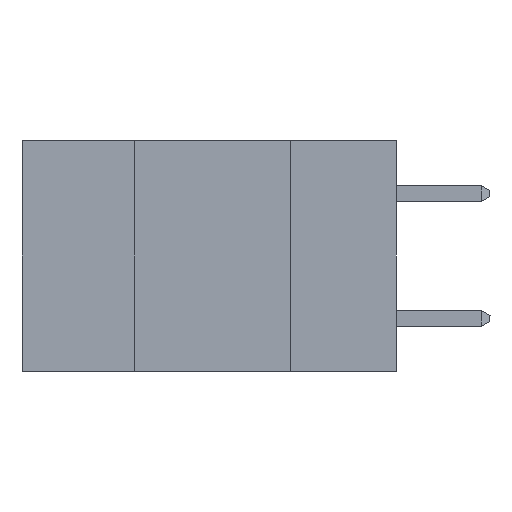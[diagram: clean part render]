
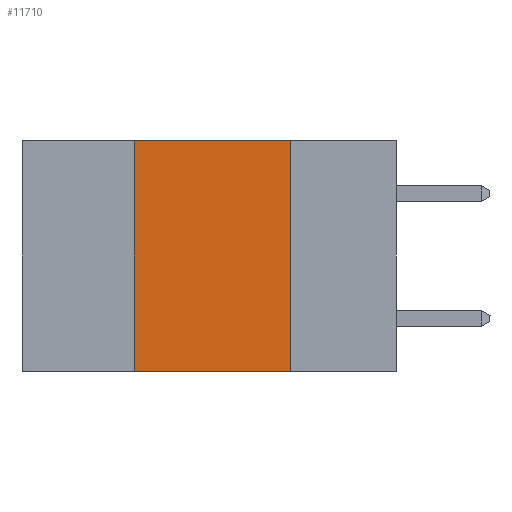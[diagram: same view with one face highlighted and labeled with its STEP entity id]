
A CAD part, left-side view. The second image highlights one B-rep face of the part: STEP entity #11710.
In plain terms, the highlighted planar face has unit normal (-1, 0, 0).
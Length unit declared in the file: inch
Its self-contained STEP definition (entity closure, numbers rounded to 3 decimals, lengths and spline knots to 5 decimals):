
#12 = ORIENTED_EDGE ( 'NONE', *, *, #7438, .F. ) ;
#440 = VECTOR ( 'NONE', #2765, 39.37008 ) ;
#784 = CARTESIAN_POINT ( 'NONE',  ( 0., 0.42, -0.37 ) ) ;
#916 = VECTOR ( 'NONE', #6709, 39.37008 ) ;
#1536 = CARTESIAN_POINT ( 'NONE',  ( 0., 0.6, 0. ) ) ;
#1639 = VERTEX_POINT ( 'NONE', #2830 ) ;
#1714 = CARTESIAN_POINT ( 'NONE',  ( 0., 0.42, -0.37 ) ) ;
#2765 = DIRECTION ( 'NONE',  ( 0., -1., 0. ) ) ;
#2816 = EDGE_CURVE ( 'NONE', #12401, #12065, #6051, .T. ) ;
#2830 = CARTESIAN_POINT ( 'NONE',  ( 0., 0.42, 0. ) ) ;
#3288 = CARTESIAN_POINT ( 'NONE',  ( 0., 0.17, -0.37 ) ) ;
#3480 = EDGE_CURVE ( 'NONE', #12401, #1639, #8670, .T. ) ;
#4676 = LINE ( 'NONE', #3288, #11927 ) ;
#4824 = VECTOR ( 'NONE', #9971, 39.37008 ) ;
#4964 = EDGE_LOOP ( 'NONE', ( #7771, #12, #9336, #8425 ) ) ;
#5524 = DIRECTION ( 'NONE',  ( 1., 0., 0. ) ) ;
#6051 = LINE ( 'NONE', #8593, #440 ) ;
#6123 = CARTESIAN_POINT ( 'NONE',  ( 0., 0.17, -0.37 ) ) ;
#6709 = DIRECTION ( 'NONE',  ( 0., 0., 1. ) ) ;
#6818 = EDGE_CURVE ( 'NONE', #8084, #12065, #4676, .T. ) ;
#7227 = DIRECTION ( 'NONE',  ( 0., 0., -1. ) ) ;
#7394 = FACE_OUTER_BOUND ( 'NONE', #4964, .T. ) ;
#7438 = EDGE_CURVE ( 'NONE', #1639, #8084, #12317, .T. ) ;
#7771 = ORIENTED_EDGE ( 'NONE', *, *, #6818, .F. ) ;
#8084 = VERTEX_POINT ( 'NONE', #9147 ) ;
#8107 = CARTESIAN_POINT ( 'NONE',  ( 0., 0.6, 0. ) ) ;
#8425 = ORIENTED_EDGE ( 'NONE', *, *, #2816, .T. ) ;
#8593 = CARTESIAN_POINT ( 'NONE',  ( 0., 0.6, -0.37 ) ) ;
#8670 = LINE ( 'NONE', #784, #916 ) ;
#9147 = CARTESIAN_POINT ( 'NONE',  ( 0., 0.17, 0. ) ) ;
#9336 = ORIENTED_EDGE ( 'NONE', *, *, #3480, .F. ) ;
#9971 = DIRECTION ( 'NONE',  ( 0., -1., 0. ) ) ;
#11138 = PLANE ( 'NONE',  #12113 ) ;
#11710 = ADVANCED_FACE ( 'NONE', ( #7394 ), #11138, .F. ) ;
#11927 = VECTOR ( 'NONE', #7227, 39.37008 ) ;
#12038 = DIRECTION ( 'NONE',  ( 0., 0., -1. ) ) ;
#12065 = VERTEX_POINT ( 'NONE', #6123 ) ;
#12113 = AXIS2_PLACEMENT_3D ( 'NONE', #1536, #5524, #12038 ) ;
#12317 = LINE ( 'NONE', #8107, #4824 ) ;
#12401 = VERTEX_POINT ( 'NONE', #1714 ) ;
